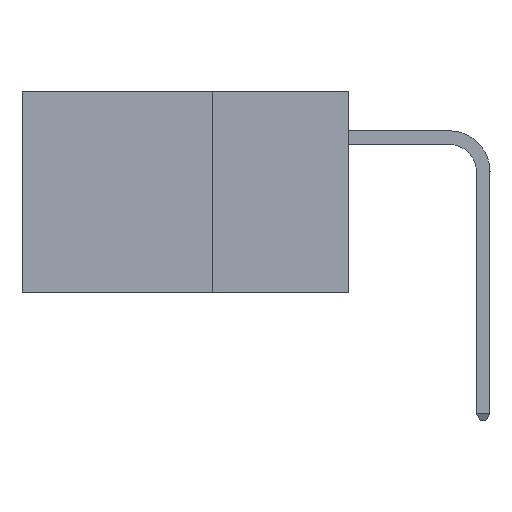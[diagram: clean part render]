
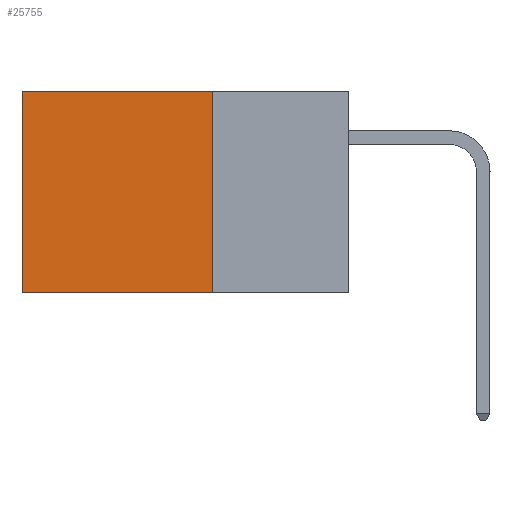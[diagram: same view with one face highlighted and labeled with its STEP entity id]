
A CAD part, left-side view. The second image highlights one B-rep face of the part: STEP entity #25755.
In plain terms, the highlighted planar face has unit normal (-1, 0, 0).
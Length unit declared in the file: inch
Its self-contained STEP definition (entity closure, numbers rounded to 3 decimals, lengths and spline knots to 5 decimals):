
#789 = ORIENTED_EDGE ( 'NONE', *, *, #16034, .T. ) ;
#1383 = CARTESIAN_POINT ( 'NONE',  ( 0.2875, 0.25, -0.37 ) ) ;
#2182 = CARTESIAN_POINT ( 'NONE',  ( 0.2875, 0.6, 0. ) ) ;
#2891 = VERTEX_POINT ( 'NONE', #2182 ) ;
#3879 = LINE ( 'NONE', #6805, #10541 ) ;
#5401 = LINE ( 'NONE', #10450, #25198 ) ;
#6805 = CARTESIAN_POINT ( 'NONE',  ( 0.2875, 0.25, 0. ) ) ;
#7740 = CARTESIAN_POINT ( 'NONE',  ( 0.2875, 0.25, 0. ) ) ;
#9703 = VECTOR ( 'NONE', #32362, 39.37008 ) ;
#10450 = CARTESIAN_POINT ( 'NONE',  ( 0.2875, 0.25, -0.37 ) ) ;
#10541 = VECTOR ( 'NONE', #18036, 39.37008 ) ;
#10602 = DIRECTION ( 'NONE',  ( 1., 0., 0. ) ) ;
#10879 = ORIENTED_EDGE ( 'NONE', *, *, #22693, .F. ) ;
#11448 = CARTESIAN_POINT ( 'NONE',  ( 0.2875, 0.6, -0.37 ) ) ;
#12046 = DIRECTION ( 'NONE',  ( 0., 0., -1. ) ) ;
#12776 = CARTESIAN_POINT ( 'NONE',  ( 0.2875, 0.6, 0. ) ) ;
#16034 = EDGE_CURVE ( 'NONE', #2891, #22567, #23734, .T. ) ;
#17703 = EDGE_LOOP ( 'NONE', ( #789, #18160, #10879, #23533 ) ) ;
#18036 = DIRECTION ( 'NONE',  ( 0., 1., 0. ) ) ;
#18160 = ORIENTED_EDGE ( 'NONE', *, *, #24349, .F. ) ;
#18720 = VERTEX_POINT ( 'NONE', #19816 ) ;
#19816 = CARTESIAN_POINT ( 'NONE',  ( 0.2875, 0.25, 0. ) ) ;
#21406 = VECTOR ( 'NONE', #12046, 39.37008 ) ;
#21523 = EDGE_CURVE ( 'NONE', #18720, #2891, #3879, .T. ) ;
#22567 = VERTEX_POINT ( 'NONE', #11448 ) ;
#22693 = EDGE_CURVE ( 'NONE', #18720, #33722, #35377, .T. ) ;
#22980 = FACE_OUTER_BOUND ( 'NONE', #17703, .T. ) ;
#23533 = ORIENTED_EDGE ( 'NONE', *, *, #21523, .T. ) ;
#23734 = LINE ( 'NONE', #12776, #9703 ) ;
#24349 = EDGE_CURVE ( 'NONE', #33722, #22567, #5401, .T. ) ;
#24533 = DIRECTION ( 'NONE',  ( 0., 1., 0. ) ) ;
#24560 = PLANE ( 'NONE',  #35895 ) ;
#25198 = VECTOR ( 'NONE', #24533, 39.37008 ) ;
#25755 = ADVANCED_FACE ( 'NONE', ( #22980 ), #24560, .F. ) ;
#28862 = CARTESIAN_POINT ( 'NONE',  ( 0.2875, 0.25, 0. ) ) ;
#30205 = DIRECTION ( 'NONE',  ( 0., 0., -1. ) ) ;
#32362 = DIRECTION ( 'NONE',  ( 0., 0., -1. ) ) ;
#33722 = VERTEX_POINT ( 'NONE', #1383 ) ;
#35377 = LINE ( 'NONE', #28862, #21406 ) ;
#35895 = AXIS2_PLACEMENT_3D ( 'NONE', #7740, #10602, #30205 ) ;
